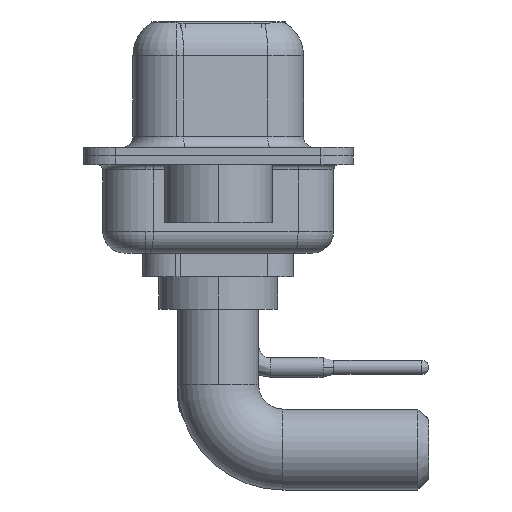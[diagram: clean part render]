
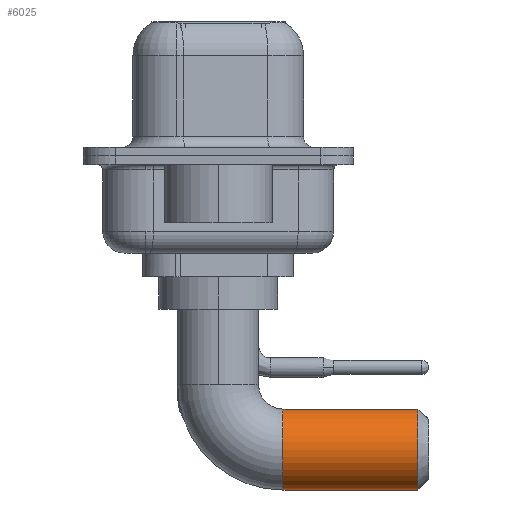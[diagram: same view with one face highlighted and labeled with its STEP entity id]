
A CAD part, left-side view. The second image highlights one B-rep face of the part: STEP entity #6025.
In plain terms, the highlighted cylindrical face has radius 1.875 mm (diameter 3.75 mm), a partial arc.
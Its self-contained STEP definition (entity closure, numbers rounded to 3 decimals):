
#1267 = LINE ( 'NONE', #4538, #6875 ) ;
#2136 = DIRECTION ( 'NONE',  ( 0., -1., 0. ) ) ;
#3393 = VERTEX_POINT ( 'NONE', #8603 ) ;
#3430 = CARTESIAN_POINT ( 'NONE',  ( 0., -9.25, -6.5 ) ) ;
#3820 = DIRECTION ( 'NONE',  ( -1., 0., 0. ) ) ;
#4538 = CARTESIAN_POINT ( 'NONE',  ( 0., -3., -4.625 ) ) ;
#4639 = DIRECTION ( 'NONE',  ( 0., -1., 0. ) ) ;
#5028 = EDGE_CURVE ( 'NONE', #7362, #3393, #10122, .T. ) ;
#5175 = AXIS2_PLACEMENT_3D ( 'NONE', #3430, #14463, #18852 ) ;
#6025 = ADVANCED_FACE ( 'NONE', ( #12867 ), #19080, .T. ) ;
#6298 = AXIS2_PLACEMENT_3D ( 'NONE', #11579, #17826, #3820 ) ;
#6357 = EDGE_CURVE ( 'NONE', #3393, #9351, #12338, .T. ) ;
#6875 = VECTOR ( 'NONE', #4639, 1000. ) ;
#7362 = VERTEX_POINT ( 'NONE', #7428 ) ;
#7428 = CARTESIAN_POINT ( 'NONE',  ( 0., -3., -8.375 ) ) ;
#7984 = ORIENTED_EDGE ( 'NONE', *, *, #9765, .F. ) ;
#8357 = DIRECTION ( 'NONE',  ( 0., 0., -1. ) ) ;
#8403 = AXIS2_PLACEMENT_3D ( 'NONE', #11113, #2136, #8357 ) ;
#8603 = CARTESIAN_POINT ( 'NONE',  ( 0., -9.25, -8.375 ) ) ;
#8958 = ORIENTED_EDGE ( 'NONE', *, *, #5028, .T. ) ;
#9351 = VERTEX_POINT ( 'NONE', #15668 ) ;
#9765 = EDGE_CURVE ( 'NONE', #14617, #9351, #1267, .T. ) ;
#10122 = LINE ( 'NONE', #16248, #13125 ) ;
#11113 = CARTESIAN_POINT ( 'NONE',  ( 0., -3., -6.5 ) ) ;
#11579 = CARTESIAN_POINT ( 'NONE',  ( 0., -3., -6.5 ) ) ;
#12338 = CIRCLE ( 'NONE', #5175, 1.875 ) ;
#12400 = ORIENTED_EDGE ( 'NONE', *, *, #6357, .T. ) ;
#12490 = EDGE_CURVE ( 'NONE', #14617, #7362, #12790, .T. ) ;
#12790 = CIRCLE ( 'NONE', #6298, 1.875 ) ;
#12867 = FACE_OUTER_BOUND ( 'NONE', #17179, .T. ) ;
#13125 = VECTOR ( 'NONE', #14818, 1000. ) ;
#14463 = DIRECTION ( 'NONE',  ( 0., 1., 0. ) ) ;
#14617 = VERTEX_POINT ( 'NONE', #17872 ) ;
#14818 = DIRECTION ( 'NONE',  ( 0., -1., 0. ) ) ;
#15668 = CARTESIAN_POINT ( 'NONE',  ( 0., -9.25, -4.625 ) ) ;
#15906 = ORIENTED_EDGE ( 'NONE', *, *, #12490, .T. ) ;
#16248 = CARTESIAN_POINT ( 'NONE',  ( 0., -3., -8.375 ) ) ;
#17179 = EDGE_LOOP ( 'NONE', ( #7984, #15906, #8958, #12400 ) ) ;
#17826 = DIRECTION ( 'NONE',  ( 0., -1., 0. ) ) ;
#17872 = CARTESIAN_POINT ( 'NONE',  ( 0., -3., -4.625 ) ) ;
#18852 = DIRECTION ( 'NONE',  ( 0., 0., -1. ) ) ;
#19080 = CYLINDRICAL_SURFACE ( 'NONE', #8403, 1.875 ) ;
